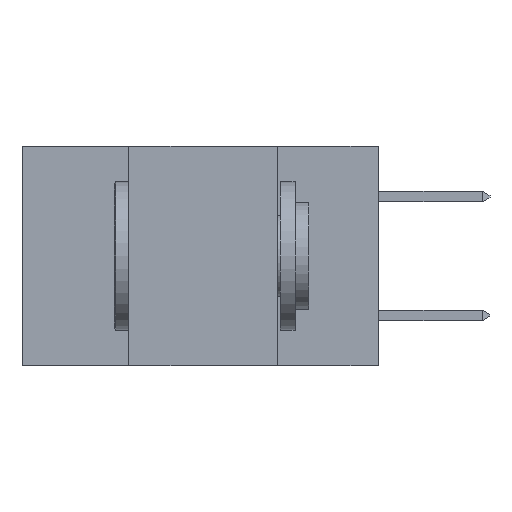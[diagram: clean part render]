
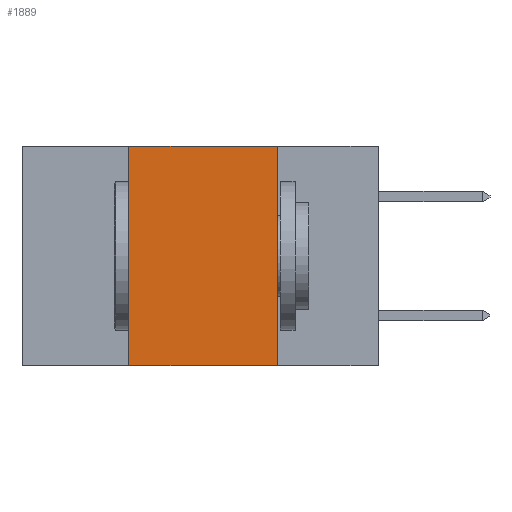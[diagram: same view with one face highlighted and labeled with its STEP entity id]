
A CAD part, left-side view. The second image highlights one B-rep face of the part: STEP entity #1889.
In plain terms, the highlighted planar face has unit normal (-1, 0, 0).
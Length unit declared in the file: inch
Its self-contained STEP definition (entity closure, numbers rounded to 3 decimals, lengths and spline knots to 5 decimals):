
#599 = EDGE_CURVE ( 'NONE', #16767, #9517, #12575, .T. ) ;
#738 = EDGE_CURVE ( 'NONE', #9517, #15961, #4556, .T. ) ;
#1889 = ADVANCED_FACE ( 'NONE', ( #3926 ), #14725, .F. ) ;
#1977 = LINE ( 'NONE', #14905, #12108 ) ;
#3346 = CARTESIAN_POINT ( 'NONE',  ( 0., 0.17, -0.37 ) ) ;
#3554 = CARTESIAN_POINT ( 'NONE',  ( 0., 0.42, -0.37 ) ) ;
#3709 = VECTOR ( 'NONE', #7555, 39.37008 ) ;
#3926 = FACE_OUTER_BOUND ( 'NONE', #15430, .T. ) ;
#4556 = LINE ( 'NONE', #19101, #19049 ) ;
#5488 = DIRECTION ( 'NONE',  ( 0., -1., 0. ) ) ;
#7198 = CARTESIAN_POINT ( 'NONE',  ( 0., 0.17, 0. ) ) ;
#7339 = ORIENTED_EDGE ( 'NONE', *, *, #22738, .F. ) ;
#7468 = DIRECTION ( 'NONE',  ( 0., -1., 0. ) ) ;
#7490 = VECTOR ( 'NONE', #7468, 39.37008 ) ;
#7555 = DIRECTION ( 'NONE',  ( 0., 0., 1. ) ) ;
#9517 = VERTEX_POINT ( 'NONE', #7198 ) ;
#10558 = VERTEX_POINT ( 'NONE', #3554 ) ;
#12030 = CARTESIAN_POINT ( 'NONE',  ( 0., 0.42, 0. ) ) ;
#12108 = VECTOR ( 'NONE', #5488, 39.37008 ) ;
#12575 = LINE ( 'NONE', #18225, #7490 ) ;
#13037 = ORIENTED_EDGE ( 'NONE', *, *, #21495, .T. ) ;
#13234 = LINE ( 'NONE', #20887, #3709 ) ;
#13465 = DIRECTION ( 'NONE',  ( 0., 0., -1. ) ) ;
#14725 = PLANE ( 'NONE',  #23523 ) ;
#14799 = CARTESIAN_POINT ( 'NONE',  ( 0., 0.6, 0. ) ) ;
#14905 = CARTESIAN_POINT ( 'NONE',  ( 0., 0.6, -0.37 ) ) ;
#15360 = DIRECTION ( 'NONE',  ( 0., 0., -1. ) ) ;
#15430 = EDGE_LOOP ( 'NONE', ( #21001, #23574, #7339, #13037 ) ) ;
#15961 = VERTEX_POINT ( 'NONE', #3346 ) ;
#16767 = VERTEX_POINT ( 'NONE', #12030 ) ;
#18225 = CARTESIAN_POINT ( 'NONE',  ( 0., 0.6, 0. ) ) ;
#19049 = VECTOR ( 'NONE', #13465, 39.37008 ) ;
#19101 = CARTESIAN_POINT ( 'NONE',  ( 0., 0.17, 0. ) ) ;
#19265 = DIRECTION ( 'NONE',  ( 1., 0., 0. ) ) ;
#20887 = CARTESIAN_POINT ( 'NONE',  ( 0., 0.42, 0. ) ) ;
#21001 = ORIENTED_EDGE ( 'NONE', *, *, #738, .F. ) ;
#21495 = EDGE_CURVE ( 'NONE', #10558, #15961, #1977, .T. ) ;
#22738 = EDGE_CURVE ( 'NONE', #10558, #16767, #13234, .T. ) ;
#23523 = AXIS2_PLACEMENT_3D ( 'NONE', #14799, #19265, #15360 ) ;
#23574 = ORIENTED_EDGE ( 'NONE', *, *, #599, .F. ) ;
